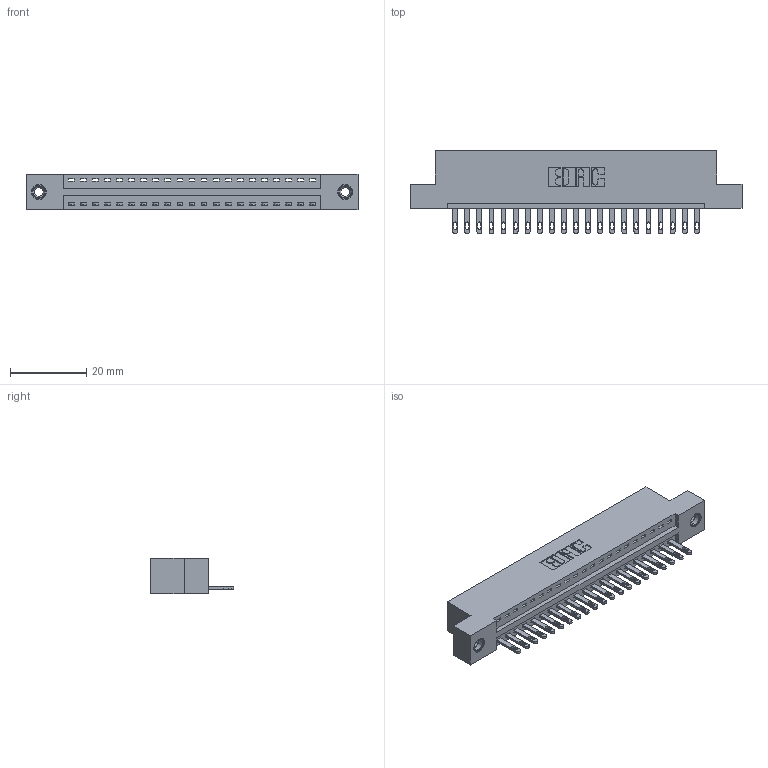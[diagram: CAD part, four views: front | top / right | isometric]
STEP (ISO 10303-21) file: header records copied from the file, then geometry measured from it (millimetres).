
FILE_DESCRIPTION (( 'STEP AP203' ), '1' );
FILE_NAME ('346-021-500-108.STEP', '2022-05-05T17:25:51', ( '' ), ( '' ), 'SwSTEP 2.0', 'SolidWorks 2020', '' );
FILE_SCHEMA (( 'CONFIG_CONTROL_DESIGN' ));
Length unit declared in the file: inch
Products named in the file (4): 345-292-001_345-293-100; 345-250-001_345-250-003-102; 346 Part_Flush Mounting Lugs - 0.156 Dia-TI; 346-021-500-108
Assembly tree (24 placements, depth 2):
  346-021-500-108
    346 Part_Flush Mounting Lugs - 0.156 Dia-TI
    345-292-001_345-293-100  x21
    345-250-001_345-250-003-102  x2
Bounding box: 87.25 x 21.84 x 9.4 mm (x, y, z)
Volume: 8213.5 mm3; surface area: 10109.9 mm2
Topology: 24 solids, 24 shells, 1316 faces, 3993 edges, 2654 vertices
Faces by surface type: plane 822, cylinder 478, cone 12, torus 4
Entity records: 16976 total; most frequent: CARTESIAN_POINT 2898, ORIENTED_EDGE 2846, DIRECTION 2611, EDGE_CURVE 1423, LINE 1183, VECTOR 1183, VERTEX_POINT 944, AXIS2_PLACEMENT_3D 714
